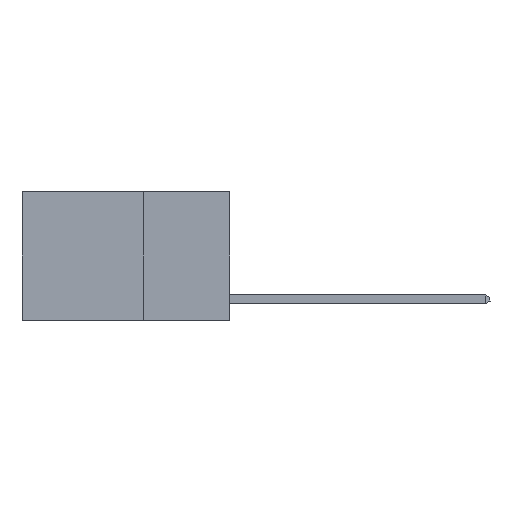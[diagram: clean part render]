
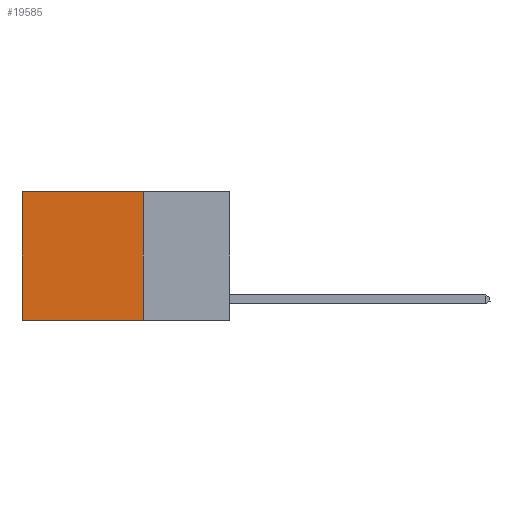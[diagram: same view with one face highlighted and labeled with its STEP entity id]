
A CAD part, left-side view. The second image highlights one B-rep face of the part: STEP entity #19585.
In plain terms, the highlighted planar face has unit normal (-1, 0, 0).
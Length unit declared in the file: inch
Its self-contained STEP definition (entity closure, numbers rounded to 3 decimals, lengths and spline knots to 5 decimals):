
#104 = EDGE_LOOP ( 'NONE', ( #613, #18353, #13572, #11493 ) ) ;
#613 = ORIENTED_EDGE ( 'NONE', *, *, #18579, .T. ) ;
#1304 = CARTESIAN_POINT ( 'NONE',  ( 0.2625, 0.25, 0. ) ) ;
#1800 = EDGE_CURVE ( 'NONE', #18133, #16577, #16754, .T. ) ;
#2557 = CARTESIAN_POINT ( 'NONE',  ( 0.2625, 0.6, -0.37 ) ) ;
#2613 = DIRECTION ( 'NONE',  ( 1., 0., 0. ) ) ;
#3128 = DIRECTION ( 'NONE',  ( 0., 1., 0. ) ) ;
#5874 = DIRECTION ( 'NONE',  ( 0., 0., -1. ) ) ;
#7548 = CARTESIAN_POINT ( 'NONE',  ( 0.2625, 0.6, 0. ) ) ;
#7590 = LINE ( 'NONE', #16297, #7634 ) ;
#7634 = VECTOR ( 'NONE', #5874, 39.37008 ) ;
#9582 = PLANE ( 'NONE',  #18298 ) ;
#10999 = VERTEX_POINT ( 'NONE', #7548 ) ;
#11493 = ORIENTED_EDGE ( 'NONE', *, *, #14627, .T. ) ;
#13411 = CARTESIAN_POINT ( 'NONE',  ( 0.2625, 0.25, -0.37 ) ) ;
#13469 = DIRECTION ( 'NONE',  ( 0., 0., -1. ) ) ;
#13572 = ORIENTED_EDGE ( 'NONE', *, *, #1800, .F. ) ;
#13719 = CARTESIAN_POINT ( 'NONE',  ( 0.2625, 0.25, 0. ) ) ;
#14066 = VECTOR ( 'NONE', #3128, 39.37008 ) ;
#14536 = VERTEX_POINT ( 'NONE', #2557 ) ;
#14627 = EDGE_CURVE ( 'NONE', #18133, #10999, #18709, .T. ) ;
#16297 = CARTESIAN_POINT ( 'NONE',  ( 0.2625, 0.6, 0. ) ) ;
#16464 = FACE_OUTER_BOUND ( 'NONE', #104, .T. ) ;
#16577 = VERTEX_POINT ( 'NONE', #20474 ) ;
#16754 = LINE ( 'NONE', #1304, #18927 ) ;
#17500 = EDGE_CURVE ( 'NONE', #16577, #14536, #20316, .T. ) ;
#18133 = VERTEX_POINT ( 'NONE', #13719 ) ;
#18298 = AXIS2_PLACEMENT_3D ( 'NONE', #20147, #2613, #13469 ) ;
#18353 = ORIENTED_EDGE ( 'NONE', *, *, #17500, .F. ) ;
#18579 = EDGE_CURVE ( 'NONE', #10999, #14536, #7590, .T. ) ;
#18709 = LINE ( 'NONE', #22372, #14066 ) ;
#18917 = VECTOR ( 'NONE', #20538, 39.37008 ) ;
#18927 = VECTOR ( 'NONE', #20328, 39.37008 ) ;
#19585 = ADVANCED_FACE ( 'NONE', ( #16464 ), #9582, .F. ) ;
#20147 = CARTESIAN_POINT ( 'NONE',  ( 0.2625, 0.25, 0. ) ) ;
#20316 = LINE ( 'NONE', #13411, #18917 ) ;
#20328 = DIRECTION ( 'NONE',  ( 0., 0., -1. ) ) ;
#20474 = CARTESIAN_POINT ( 'NONE',  ( 0.2625, 0.25, -0.37 ) ) ;
#20538 = DIRECTION ( 'NONE',  ( 0., 1., 0. ) ) ;
#22372 = CARTESIAN_POINT ( 'NONE',  ( 0.2625, 0.25, 0. ) ) ;
